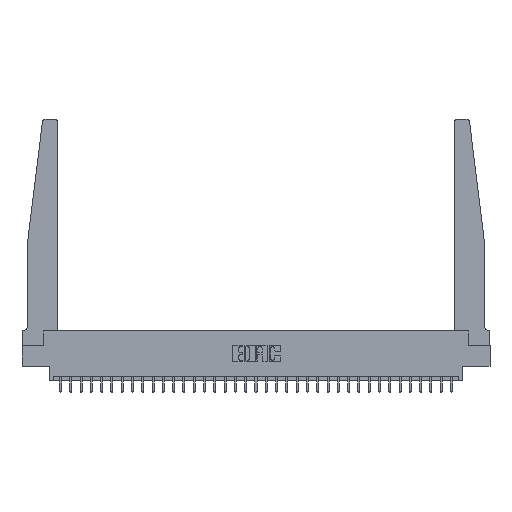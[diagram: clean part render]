
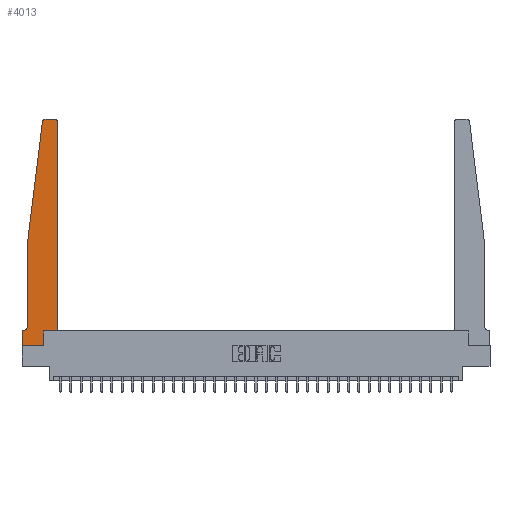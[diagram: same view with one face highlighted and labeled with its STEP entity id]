
A CAD part, top view. The second image highlights one B-rep face of the part: STEP entity #4013.
In plain terms, the highlighted planar face has unit normal (0, 0, 1).
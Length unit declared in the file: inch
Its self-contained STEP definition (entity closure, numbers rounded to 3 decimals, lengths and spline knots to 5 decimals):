
#534 = VERTEX_POINT ( 'NONE', #2431 ) ;
#626 = DIRECTION ( 'NONE',  ( -0.122, -0.992, 0. ) ) ;
#758 = CARTESIAN_POINT ( 'NONE',  ( 0.2605, 0.18, 0.37 ) ) ;
#1263 = CARTESIAN_POINT ( 'NONE',  ( 0.25, 2.75, 0.37 ) ) ;
#1660 = DIRECTION ( 'NONE',  ( 1., 0., 0. ) ) ;
#2289 = DIRECTION ( 'NONE',  ( -1., 0., 0. ) ) ;
#2404 = CIRCLE ( 'NONE', #12895, 0.05 ) ;
#2431 = CARTESIAN_POINT ( 'NONE',  ( 0.425, 0.18, 0.37 ) ) ;
#2962 = VERTEX_POINT ( 'NONE', #15942 ) ;
#2987 = CIRCLE ( 'NONE', #24600, 0.03 ) ;
#3501 = VECTOR ( 'NONE', #9354, 39.37008 ) ;
#4013 = ADVANCED_FACE ( 'NONE', ( #28829 ), #10802, .T. ) ;
#4204 = CARTESIAN_POINT ( 'NONE',  ( 0., 0., 0.37 ) ) ;
#4511 = VERTEX_POINT ( 'NONE', #12360 ) ;
#4556 = CARTESIAN_POINT ( 'NONE',  ( 0.425, 2.72, 0.37 ) ) ;
#6033 = CARTESIAN_POINT ( 'NONE',  ( 0.425, 0.18, 0.37 ) ) ;
#6043 = VECTOR ( 'NONE', #27687, 39.37008 ) ;
#6764 = DIRECTION ( 'NONE',  ( 0., -1., 0. ) ) ;
#6953 = CARTESIAN_POINT ( 'NONE',  ( 0.065, 0.1875, 0.37 ) ) ;
#8228 = CARTESIAN_POINT ( 'NONE',  ( 0., 0.1875, 0.37 ) ) ;
#8427 = DIRECTION ( 'NONE',  ( 0., 1., 0. ) ) ;
#8445 = EDGE_CURVE ( 'NONE', #534, #17885, #30395, .T. ) ;
#9354 = DIRECTION ( 'NONE',  ( 1., 0., 0. ) ) ;
#9424 = LINE ( 'NONE', #6953, #22095 ) ;
#9675 = EDGE_CURVE ( 'NONE', #17100, #22207, #22933, .T. ) ;
#9902 = EDGE_CURVE ( 'NONE', #19322, #17100, #29567, .T. ) ;
#10493 = CARTESIAN_POINT ( 'NONE',  ( 0.24675, 2.72367, 0.37 ) ) ;
#10646 = VECTOR ( 'NONE', #25573, 39.37008 ) ;
#10802 = PLANE ( 'NONE',  #22523 ) ;
#10873 = EDGE_CURVE ( 'NONE', #22207, #534, #23235, .T. ) ;
#11099 = CARTESIAN_POINT ( 'NONE',  ( 0., 0., 0.37 ) ) ;
#11155 = VERTEX_POINT ( 'NONE', #15362 ) ;
#11506 = DIRECTION ( 'NONE',  ( 0., 0., -1. ) ) ;
#11644 = CARTESIAN_POINT ( 'NONE',  ( 0.425, 0.18, 0.37 ) ) ;
#11864 = CARTESIAN_POINT ( 'NONE',  ( 0.27653, 2.72, 0.37 ) ) ;
#12202 = VECTOR ( 'NONE', #8427, 39.37008 ) ;
#12360 = CARTESIAN_POINT ( 'NONE',  ( 0.015, 0.1875, 0.37 ) ) ;
#12784 = CARTESIAN_POINT ( 'NONE',  ( 0.2605, 0., 0.37 ) ) ;
#12895 = AXIS2_PLACEMENT_3D ( 'NONE', #25694, #11506, #28115 ) ;
#13052 = LINE ( 'NONE', #14924, #19412 ) ;
#14227 = DIRECTION ( 'NONE',  ( 1., 0., 0. ) ) ;
#14849 = LINE ( 'NONE', #21048, #27489 ) ;
#14924 = CARTESIAN_POINT ( 'NONE',  ( 0.065, 1.25, 0.37 ) ) ;
#15272 = EDGE_CURVE ( 'NONE', #20879, #4511, #2404, .T. ) ;
#15362 = CARTESIAN_POINT ( 'NONE',  ( 0.395, 2.75, 0.37 ) ) ;
#15575 = DIRECTION ( 'NONE',  ( 1., 0., 0. ) ) ;
#15926 = DIRECTION ( 'NONE',  ( 0., 0., 1. ) ) ;
#15942 = CARTESIAN_POINT ( 'NONE',  ( 0.065, 1.25, 0.37 ) ) ;
#16018 = ORIENTED_EDGE ( 'NONE', *, *, #23061, .T. ) ;
#16047 = ORIENTED_EDGE ( 'NONE', *, *, #26193, .T. ) ;
#16355 = ORIENTED_EDGE ( 'NONE', *, *, #22851, .T. ) ;
#16464 = ORIENTED_EDGE ( 'NONE', *, *, #23934, .T. ) ;
#16492 = ORIENTED_EDGE ( 'NONE', *, *, #15272, .T. ) ;
#16595 = VECTOR ( 'NONE', #17846, 39.37008 ) ;
#16873 = ORIENTED_EDGE ( 'NONE', *, *, #21606, .T. ) ;
#16952 = ORIENTED_EDGE ( 'NONE', *, *, #28624, .T. ) ;
#17100 = VERTEX_POINT ( 'NONE', #12784 ) ;
#17141 = VERTEX_POINT ( 'NONE', #8228 ) ;
#17263 = ORIENTED_EDGE ( 'NONE', *, *, #9902, .T. ) ;
#17536 = VERTEX_POINT ( 'NONE', #23874 ) ;
#17696 = ORIENTED_EDGE ( 'NONE', *, *, #9675, .T. ) ;
#17794 = ORIENTED_EDGE ( 'NONE', *, *, #10873, .T. ) ;
#17846 = DIRECTION ( 'NONE',  ( 0., 1., 0. ) ) ;
#17885 = VERTEX_POINT ( 'NONE', #4556 ) ;
#18070 = ORIENTED_EDGE ( 'NONE', *, *, #8445, .T. ) ;
#18106 = ORIENTED_EDGE ( 'NONE', *, *, #29222, .T. ) ;
#19322 = VERTEX_POINT ( 'NONE', #27016 ) ;
#19412 = VECTOR ( 'NONE', #626, 39.37008 ) ;
#19455 = LINE ( 'NONE', #11099, #6043 ) ;
#19785 = VECTOR ( 'NONE', #22834, 39.37008 ) ;
#20879 = VERTEX_POINT ( 'NONE', #23340 ) ;
#21048 = CARTESIAN_POINT ( 'NONE',  ( 0.065, 1.25, 0.37 ) ) ;
#21606 = EDGE_CURVE ( 'NONE', #4511, #17141, #9424, .T. ) ;
#21816 = VERTEX_POINT ( 'NONE', #10493 ) ;
#21888 = EDGE_LOOP ( 'NONE', ( #16018, #16047, #16355, #16464, #16492, #16873, #16952, #17263, #17696, #17794, #18070, #18106 ) ) ;
#22095 = VECTOR ( 'NONE', #2289, 39.37008 ) ;
#22207 = VERTEX_POINT ( 'NONE', #758 ) ;
#22523 = AXIS2_PLACEMENT_3D ( 'NONE', #27401, #29765, #15575 ) ;
#22834 = DIRECTION ( 'NONE',  ( -1., 0., 0. ) ) ;
#22851 = EDGE_CURVE ( 'NONE', #21816, #2962, #13052, .T. ) ;
#22933 = LINE ( 'NONE', #24865, #16595 ) ;
#23061 = EDGE_CURVE ( 'NONE', #11155, #17536, #26021, .T. ) ;
#23235 = LINE ( 'NONE', #11644, #3501 ) ;
#23340 = CARTESIAN_POINT ( 'NONE',  ( 0.065, 0.2375, 0.37 ) ) ;
#23874 = CARTESIAN_POINT ( 'NONE',  ( 0.27653, 2.75, 0.37 ) ) ;
#23934 = EDGE_CURVE ( 'NONE', #2962, #20879, #14849, .T. ) ;
#24600 = AXIS2_PLACEMENT_3D ( 'NONE', #30121, #15926, #1660 ) ;
#24865 = CARTESIAN_POINT ( 'NONE',  ( 0.2605, 0.18, 0.37 ) ) ;
#25133 = CIRCLE ( 'NONE', #26729, 0.03 ) ;
#25573 = DIRECTION ( 'NONE',  ( 1., 0., 0. ) ) ;
#25694 = CARTESIAN_POINT ( 'NONE',  ( 0.015, 0.2375, 0.37 ) ) ;
#26021 = LINE ( 'NONE', #1263, #19785 ) ;
#26193 = EDGE_CURVE ( 'NONE', #17536, #21816, #25133, .T. ) ;
#26729 = AXIS2_PLACEMENT_3D ( 'NONE', #11864, #28481, #14227 ) ;
#27016 = CARTESIAN_POINT ( 'NONE',  ( 0., 0., 0.37 ) ) ;
#27401 = CARTESIAN_POINT ( 'NONE',  ( 0., 0.1875, 0.37 ) ) ;
#27489 = VECTOR ( 'NONE', #6764, 39.37008 ) ;
#27687 = DIRECTION ( 'NONE',  ( 0., -1., 0. ) ) ;
#28115 = DIRECTION ( 'NONE',  ( -1., 0., 0. ) ) ;
#28481 = DIRECTION ( 'NONE',  ( 0., 0., 1. ) ) ;
#28624 = EDGE_CURVE ( 'NONE', #17141, #19322, #19455, .T. ) ;
#28829 = FACE_OUTER_BOUND ( 'NONE', #21888, .T. ) ;
#29222 = EDGE_CURVE ( 'NONE', #17885, #11155, #2987, .T. ) ;
#29567 = LINE ( 'NONE', #4204, #10646 ) ;
#29765 = DIRECTION ( 'NONE',  ( 0., 0., 1. ) ) ;
#30121 = CARTESIAN_POINT ( 'NONE',  ( 0.395, 2.72, 0.37 ) ) ;
#30395 = LINE ( 'NONE', #6033, #12202 ) ;
